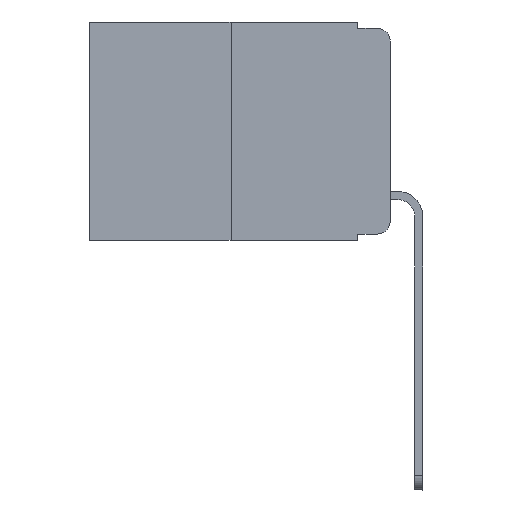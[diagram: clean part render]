
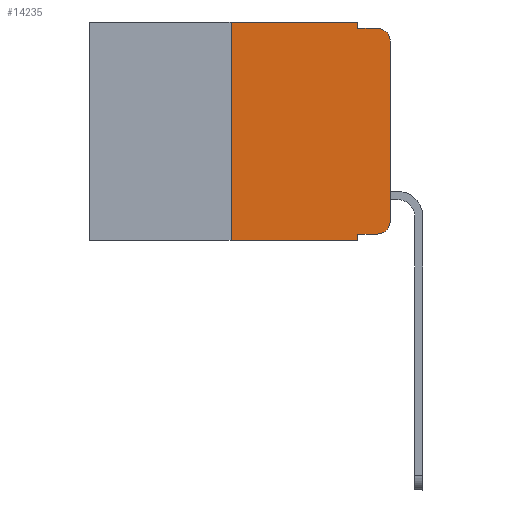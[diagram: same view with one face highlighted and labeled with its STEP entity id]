
A CAD part, left-side view. The second image highlights one B-rep face of the part: STEP entity #14235.
In plain terms, the highlighted planar face has unit normal (-1, 0, 0).
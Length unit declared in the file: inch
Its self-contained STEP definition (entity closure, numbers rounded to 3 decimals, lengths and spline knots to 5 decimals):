
#32 = CIRCLE ( 'NONE', #5936, 0.02 ) ;
#225 = DIRECTION ( 'NONE',  ( 0., 0., -1. ) ) ;
#716 = VERTEX_POINT ( 'NONE', #3678 ) ;
#1160 = LINE ( 'NONE', #21613, #8992 ) ;
#1733 = VECTOR ( 'NONE', #19836, 39.37008 ) ;
#1847 = CARTESIAN_POINT ( 'NONE',  ( 0., 0.02, -0.313 ) ) ;
#1945 = FACE_OUTER_BOUND ( 'NONE', #18271, .T. ) ;
#3289 = LINE ( 'NONE', #8831, #22703 ) ;
#3678 = CARTESIAN_POINT ( 'NONE',  ( 0., 0., -0.03 ) ) ;
#3713 = DIRECTION ( 'NONE',  ( 0., 0., -1. ) ) ;
#4138 = EDGE_CURVE ( 'NONE', #11748, #6694, #8531, .T. ) ;
#4299 = LINE ( 'NONE', #19366, #12290 ) ;
#4486 = VERTEX_POINT ( 'NONE', #10575 ) ;
#4558 = EDGE_CURVE ( 'NONE', #11748, #6860, #3289, .T. ) ;
#5009 = VECTOR ( 'NONE', #20964, 39.37008 ) ;
#5034 = LINE ( 'NONE', #14162, #1733 ) ;
#5490 = EDGE_CURVE ( 'NONE', #10599, #4486, #24320, .T. ) ;
#5534 = DIRECTION ( 'NONE',  ( -1., 0., 0. ) ) ;
#5870 = EDGE_CURVE ( 'NONE', #9044, #7548, #13250, .T. ) ;
#5936 = AXIS2_PLACEMENT_3D ( 'NONE', #13847, #9893, #12128 ) ;
#6694 = VERTEX_POINT ( 'NONE', #9623 ) ;
#6860 = VERTEX_POINT ( 'NONE', #23449 ) ;
#7283 = ORIENTED_EDGE ( 'NONE', *, *, #5870, .T. ) ;
#7440 = VERTEX_POINT ( 'NONE', #19837 ) ;
#7548 = VERTEX_POINT ( 'NONE', #15145 ) ;
#7607 = PLANE ( 'NONE',  #11544 ) ;
#7843 = EDGE_CURVE ( 'NONE', #9955, #6860, #1160, .T. ) ;
#8467 = ORIENTED_EDGE ( 'NONE', *, *, #17660, .T. ) ;
#8531 = LINE ( 'NONE', #9357, #19135 ) ;
#8831 = CARTESIAN_POINT ( 'NONE',  ( 0., 0.473, -0.343 ) ) ;
#8992 = VECTOR ( 'NONE', #19777, 39.37008 ) ;
#9044 = VERTEX_POINT ( 'NONE', #23734 ) ;
#9357 = CARTESIAN_POINT ( 'NONE',  ( 0., 0.25, 0. ) ) ;
#9623 = CARTESIAN_POINT ( 'NONE',  ( 0., 0.25, 0. ) ) ;
#9893 = DIRECTION ( 'NONE',  ( -1., 0., 0. ) ) ;
#9955 = VERTEX_POINT ( 'NONE', #15915 ) ;
#10575 = CARTESIAN_POINT ( 'NONE',  ( 0., 0.02, -0.01 ) ) ;
#10599 = VERTEX_POINT ( 'NONE', #15450 ) ;
#10815 = DIRECTION ( 'NONE',  ( 0., -1., 0. ) ) ;
#10993 = ORIENTED_EDGE ( 'NONE', *, *, #11755, .T. ) ;
#11001 = CARTESIAN_POINT ( 'NONE',  ( 0., 0.473, 0. ) ) ;
#11544 = AXIS2_PLACEMENT_3D ( 'NONE', #20790, #18950, #15501 ) ;
#11623 = ORIENTED_EDGE ( 'NONE', *, *, #23036, .F. ) ;
#11748 = VERTEX_POINT ( 'NONE', #19157 ) ;
#11755 = EDGE_CURVE ( 'NONE', #716, #4486, #32, .T. ) ;
#12113 = VECTOR ( 'NONE', #3713, 39.37008 ) ;
#12128 = DIRECTION ( 'NONE',  ( 0., 0., -1. ) ) ;
#12290 = VECTOR ( 'NONE', #15198, 39.37008 ) ;
#12451 = ORIENTED_EDGE ( 'NONE', *, *, #4558, .T. ) ;
#12715 = ORIENTED_EDGE ( 'NONE', *, *, #7843, .F. ) ;
#12892 = ORIENTED_EDGE ( 'NONE', *, *, #15851, .T. ) ;
#12967 = CARTESIAN_POINT ( 'NONE',  ( 0., 0.051, 0. ) ) ;
#13092 = LINE ( 'NONE', #12967, #12113 ) ;
#13250 = CIRCLE ( 'NONE', #20768, 0.02 ) ;
#13847 = CARTESIAN_POINT ( 'NONE',  ( 0., 0.02, -0.03 ) ) ;
#14162 = CARTESIAN_POINT ( 'NONE',  ( 0., 0., 0. ) ) ;
#14235 = ADVANCED_FACE ( 'NONE', ( #1945 ), #7607, .F. ) ;
#15145 = CARTESIAN_POINT ( 'NONE',  ( 0., 0., -0.313 ) ) ;
#15198 = DIRECTION ( 'NONE',  ( 0., -1., 0. ) ) ;
#15450 = CARTESIAN_POINT ( 'NONE',  ( 0., 0.051, -0.01 ) ) ;
#15501 = DIRECTION ( 'NONE',  ( 0., 0., -1. ) ) ;
#15851 = EDGE_CURVE ( 'NONE', #9955, #9044, #4299, .T. ) ;
#15915 = CARTESIAN_POINT ( 'NONE',  ( 0., 0.051, -0.333 ) ) ;
#16417 = ORIENTED_EDGE ( 'NONE', *, *, #5490, .F. ) ;
#17144 = CARTESIAN_POINT ( 'NONE',  ( 0., 0.051, -0.01 ) ) ;
#17660 = EDGE_CURVE ( 'NONE', #7548, #716, #5034, .T. ) ;
#18031 = DIRECTION ( 'NONE',  ( 0., 0., 1. ) ) ;
#18080 = ORIENTED_EDGE ( 'NONE', *, *, #4138, .F. ) ;
#18271 = EDGE_LOOP ( 'NONE', ( #8467, #10993, #16417, #11623, #22792, #18080, #12451, #12715, #12892, #7283 ) ) ;
#18392 = LINE ( 'NONE', #11001, #21553 ) ;
#18950 = DIRECTION ( 'NONE',  ( 1., 0., 0. ) ) ;
#19135 = VECTOR ( 'NONE', #18031, 39.37008 ) ;
#19157 = CARTESIAN_POINT ( 'NONE',  ( 0., 0.25, -0.343 ) ) ;
#19366 = CARTESIAN_POINT ( 'NONE',  ( 0., 0.051, -0.333 ) ) ;
#19777 = DIRECTION ( 'NONE',  ( 0., 0., -1. ) ) ;
#19836 = DIRECTION ( 'NONE',  ( 0., 0., 1. ) ) ;
#19837 = CARTESIAN_POINT ( 'NONE',  ( 0., 0.051, 0. ) ) ;
#20768 = AXIS2_PLACEMENT_3D ( 'NONE', #1847, #5534, #225 ) ;
#20790 = CARTESIAN_POINT ( 'NONE',  ( 0., 0.473, 0. ) ) ;
#20964 = DIRECTION ( 'NONE',  ( 0., -1., 0. ) ) ;
#21553 = VECTOR ( 'NONE', #21974, 39.37008 ) ;
#21613 = CARTESIAN_POINT ( 'NONE',  ( 0., 0.051, 0. ) ) ;
#21974 = DIRECTION ( 'NONE',  ( 0., -1., 0. ) ) ;
#22703 = VECTOR ( 'NONE', #10815, 39.37008 ) ;
#22792 = ORIENTED_EDGE ( 'NONE', *, *, #22833, .F. ) ;
#22833 = EDGE_CURVE ( 'NONE', #6694, #7440, #18392, .T. ) ;
#23036 = EDGE_CURVE ( 'NONE', #7440, #10599, #13092, .T. ) ;
#23449 = CARTESIAN_POINT ( 'NONE',  ( 0., 0.051, -0.343 ) ) ;
#23734 = CARTESIAN_POINT ( 'NONE',  ( 0., 0.02, -0.333 ) ) ;
#24320 = LINE ( 'NONE', #17144, #5009 ) ;
